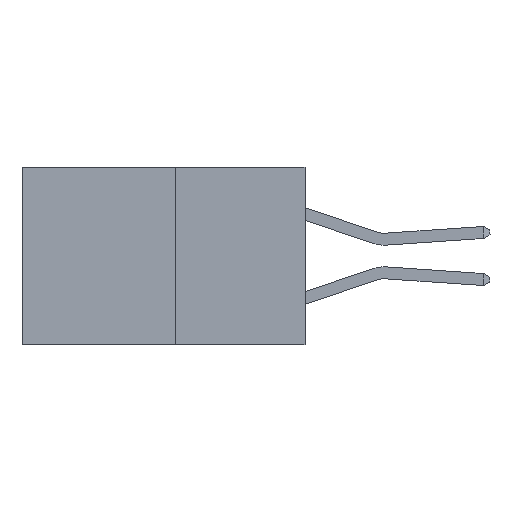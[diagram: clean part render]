
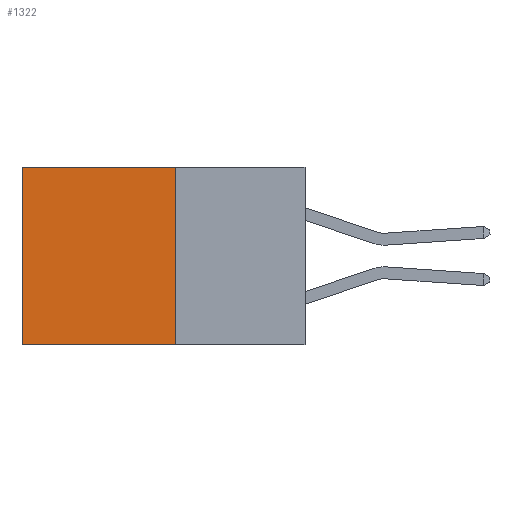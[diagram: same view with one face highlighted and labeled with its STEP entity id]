
A CAD part, left-side view. The second image highlights one B-rep face of the part: STEP entity #1322.
In plain terms, the highlighted planar face has unit normal (-1, 0, 0).
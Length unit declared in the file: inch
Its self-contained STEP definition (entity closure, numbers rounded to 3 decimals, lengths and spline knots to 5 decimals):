
#317 = PLANE ( 'NONE',  #4604 ) ;
#471 = VECTOR ( 'NONE', #2936, 39.37008 ) ;
#553 = ORIENTED_EDGE ( 'NONE', *, *, #2768, .T. ) ;
#601 = VERTEX_POINT ( 'NONE', #1639 ) ;
#635 = VECTOR ( 'NONE', #7979, 39.37008 ) ;
#949 = LINE ( 'NONE', #1488, #471 ) ;
#1059 = CARTESIAN_POINT ( 'NONE',  ( 0.277, 0.27, -0.37 ) ) ;
#1322 = ADVANCED_FACE ( 'NONE', ( #4173 ), #317, .F. ) ;
#1450 = DIRECTION ( 'NONE',  ( 0., 0., -1. ) ) ;
#1471 = CARTESIAN_POINT ( 'NONE',  ( 0.277, 0.27, -0.37 ) ) ;
#1474 = ORIENTED_EDGE ( 'NONE', *, *, #3049, .F. ) ;
#1488 = CARTESIAN_POINT ( 'NONE',  ( 0.277, 0.59, -0.37 ) ) ;
#1608 = ORIENTED_EDGE ( 'NONE', *, *, #8701, .F. ) ;
#1639 = CARTESIAN_POINT ( 'NONE',  ( 0.277, 0.59, -0.37 ) ) ;
#2304 = EDGE_LOOP ( 'NONE', ( #3151, #1608, #1474, #553 ) ) ;
#2617 = VERTEX_POINT ( 'NONE', #6386 ) ;
#2768 = EDGE_CURVE ( 'NONE', #2617, #3608, #8845, .T. ) ;
#2936 = DIRECTION ( 'NONE',  ( 0., 0., -1. ) ) ;
#2940 = CARTESIAN_POINT ( 'NONE',  ( 0.277, 0.27, -0.37 ) ) ;
#3049 = EDGE_CURVE ( 'NONE', #2617, #6818, #8516, .T. ) ;
#3151 = ORIENTED_EDGE ( 'NONE', *, *, #5017, .T. ) ;
#3608 = VERTEX_POINT ( 'NONE', #4612 ) ;
#4173 = FACE_OUTER_BOUND ( 'NONE', #2304, .T. ) ;
#4491 = LINE ( 'NONE', #1059, #635 ) ;
#4604 = AXIS2_PLACEMENT_3D ( 'NONE', #5792, #5962, #5908 ) ;
#4612 = CARTESIAN_POINT ( 'NONE',  ( 0.277, 0.59, 0. ) ) ;
#5007 = VECTOR ( 'NONE', #5057, 39.37008 ) ;
#5017 = EDGE_CURVE ( 'NONE', #3608, #601, #949, .T. ) ;
#5040 = CARTESIAN_POINT ( 'NONE',  ( 0.277, 0.27, 0. ) ) ;
#5057 = DIRECTION ( 'NONE',  ( 0., 1., 0. ) ) ;
#5792 = CARTESIAN_POINT ( 'NONE',  ( 0.277, 0.27, -0.37 ) ) ;
#5908 = DIRECTION ( 'NONE',  ( 0., 0., -1. ) ) ;
#5962 = DIRECTION ( 'NONE',  ( 1., 0., 0. ) ) ;
#6386 = CARTESIAN_POINT ( 'NONE',  ( 0.277, 0.27, 0. ) ) ;
#6818 = VERTEX_POINT ( 'NONE', #2940 ) ;
#7979 = DIRECTION ( 'NONE',  ( 0., 1., 0. ) ) ;
#8317 = VECTOR ( 'NONE', #1450, 39.37008 ) ;
#8516 = LINE ( 'NONE', #1471, #8317 ) ;
#8701 = EDGE_CURVE ( 'NONE', #6818, #601, #4491, .T. ) ;
#8845 = LINE ( 'NONE', #5040, #5007 ) ;
